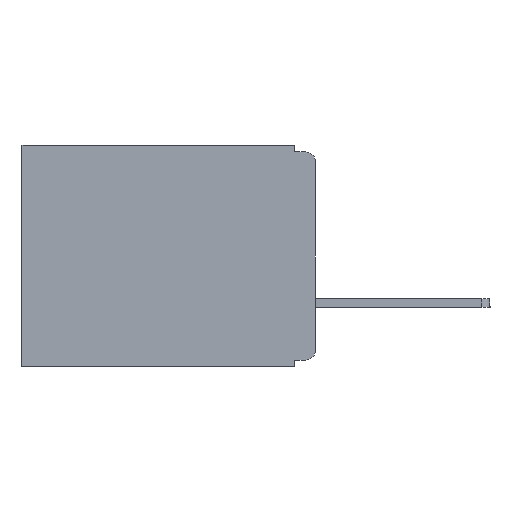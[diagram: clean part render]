
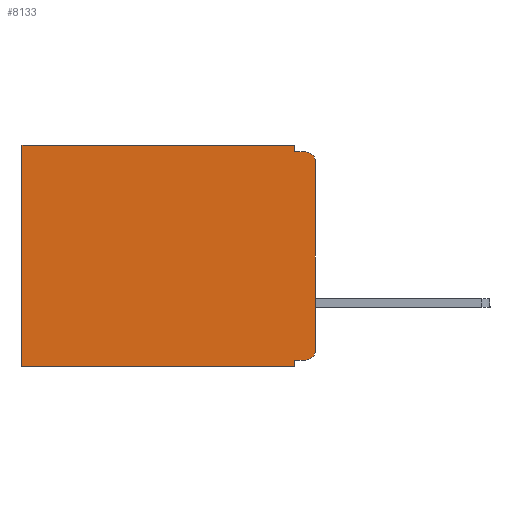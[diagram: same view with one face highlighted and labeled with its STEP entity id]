
A CAD part, left-side view. The second image highlights one B-rep face of the part: STEP entity #8133.
In plain terms, the highlighted planar face has unit normal (-1, 0, 0).
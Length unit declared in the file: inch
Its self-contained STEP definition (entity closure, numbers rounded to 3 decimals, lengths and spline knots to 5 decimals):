
#170 = CARTESIAN_POINT ( 'NONE',  ( 0.3, 0.437, -0.33 ) ) ;
#363 = CARTESIAN_POINT ( 'NONE',  ( 0.3, 0.031, -0.33 ) ) ;
#392 = CARTESIAN_POINT ( 'NONE',  ( 0.3, 0.031, 0. ) ) ;
#911 = ORIENTED_EDGE ( 'NONE', *, *, #4265, .T. ) ;
#1188 = VECTOR ( 'NONE', #18793, 39.37008 ) ;
#1235 = LINE ( 'NONE', #18116, #10656 ) ;
#1753 = DIRECTION ( 'NONE',  ( 0., 0., -1. ) ) ;
#1786 = LINE ( 'NONE', #16925, #1188 ) ;
#2096 = ORIENTED_EDGE ( 'NONE', *, *, #14630, .F. ) ;
#2279 = CARTESIAN_POINT ( 'NONE',  ( 0.3, 0.015, -0.025 ) ) ;
#2338 = CARTESIAN_POINT ( 'NONE',  ( 0.3, 0., -0.01 ) ) ;
#3538 = EDGE_CURVE ( 'NONE', #23070, #21568, #7645, .T. ) ;
#3553 = ORIENTED_EDGE ( 'NONE', *, *, #13994, .F. ) ;
#3990 = VECTOR ( 'NONE', #21921, 39.37008 ) ;
#4249 = VECTOR ( 'NONE', #19143, 39.37008 ) ;
#4265 = EDGE_CURVE ( 'NONE', #5508, #6899, #19861, .T. ) ;
#4614 = LINE ( 'NONE', #170, #9619 ) ;
#4848 = LINE ( 'NONE', #2338, #4249 ) ;
#5079 = AXIS2_PLACEMENT_3D ( 'NONE', #2279, #23373, #1753 ) ;
#5374 = EDGE_CURVE ( 'NONE', #23273, #9609, #4614, .T. ) ;
#5508 = VERTEX_POINT ( 'NONE', #17325 ) ;
#5601 = FACE_OUTER_BOUND ( 'NONE', #21836, .T. ) ;
#5902 = DIRECTION ( 'NONE',  ( 0., 0., -1. ) ) ;
#5985 = CIRCLE ( 'NONE', #12272, 0.015 ) ;
#6305 = CARTESIAN_POINT ( 'NONE',  ( 0.3, 0., -0.33 ) ) ;
#6521 = ORIENTED_EDGE ( 'NONE', *, *, #20665, .T. ) ;
#6614 = DIRECTION ( 'NONE',  ( -1., 0., 0. ) ) ;
#6899 = VERTEX_POINT ( 'NONE', #7066 ) ;
#7066 = CARTESIAN_POINT ( 'NONE',  ( 0.3, 0.015, -0.01 ) ) ;
#7314 = CARTESIAN_POINT ( 'NONE',  ( 0.3, 0.031, 0. ) ) ;
#7359 = ORIENTED_EDGE ( 'NONE', *, *, #3538, .F. ) ;
#7623 = DIRECTION ( 'NONE',  ( 0., 0., -1. ) ) ;
#7645 = LINE ( 'NONE', #392, #16981 ) ;
#7789 = CARTESIAN_POINT ( 'NONE',  ( 0.3, 0.031, -0.32 ) ) ;
#8133 = ADVANCED_FACE ( 'NONE', ( #5601 ), #17485, .F. ) ;
#8206 = DIRECTION ( 'NONE',  ( 0., 0., -1. ) ) ;
#8293 = ORIENTED_EDGE ( 'NONE', *, *, #12749, .F. ) ;
#8948 = CARTESIAN_POINT ( 'NONE',  ( 0.3, 0., 0. ) ) ;
#9609 = VERTEX_POINT ( 'NONE', #23721 ) ;
#9619 = VECTOR ( 'NONE', #7623, 39.37008 ) ;
#10656 = VECTOR ( 'NONE', #19975, 39.37008 ) ;
#11557 = CARTESIAN_POINT ( 'NONE',  ( 0.3, 0., -0.33 ) ) ;
#12272 = AXIS2_PLACEMENT_3D ( 'NONE', #17796, #6614, #19668 ) ;
#12738 = LINE ( 'NONE', #8948, #3990 ) ;
#12749 = EDGE_CURVE ( 'NONE', #16377, #22669, #16450, .T. ) ;
#13451 = EDGE_CURVE ( 'NONE', #23070, #23273, #12738, .T. ) ;
#13584 = AXIS2_PLACEMENT_3D ( 'NONE', #6305, #19371, #8206 ) ;
#13852 = VECTOR ( 'NONE', #5902, 39.37008 ) ;
#13994 = EDGE_CURVE ( 'NONE', #21568, #6899, #4848, .T. ) ;
#14432 = LINE ( 'NONE', #11557, #13852 ) ;
#14630 = EDGE_CURVE ( 'NONE', #5508, #19180, #14432, .T. ) ;
#14648 = ORIENTED_EDGE ( 'NONE', *, *, #15454, .F. ) ;
#15367 = CARTESIAN_POINT ( 'NONE',  ( 0.3, 0.437, 0. ) ) ;
#15454 = EDGE_CURVE ( 'NONE', #22669, #9609, #1235, .T. ) ;
#16316 = EDGE_CURVE ( 'NONE', #19260, #16377, #1786, .T. ) ;
#16377 = VERTEX_POINT ( 'NONE', #7789 ) ;
#16410 = ORIENTED_EDGE ( 'NONE', *, *, #5374, .T. ) ;
#16450 = LINE ( 'NONE', #18084, #21387 ) ;
#16925 = CARTESIAN_POINT ( 'NONE',  ( 0.3, 0., -0.32 ) ) ;
#16981 = VECTOR ( 'NONE', #17704, 39.37008 ) ;
#17325 = CARTESIAN_POINT ( 'NONE',  ( 0.3, 0., -0.025 ) ) ;
#17485 = PLANE ( 'NONE',  #13584 ) ;
#17704 = DIRECTION ( 'NONE',  ( 0., 0., -1. ) ) ;
#17796 = CARTESIAN_POINT ( 'NONE',  ( 0.3, 0.015, -0.305 ) ) ;
#18084 = CARTESIAN_POINT ( 'NONE',  ( 0.3, 0.031, -0.33 ) ) ;
#18116 = CARTESIAN_POINT ( 'NONE',  ( 0.3, 0., -0.33 ) ) ;
#18793 = DIRECTION ( 'NONE',  ( 0., 1., 0. ) ) ;
#19143 = DIRECTION ( 'NONE',  ( 0., -1., 0. ) ) ;
#19180 = VERTEX_POINT ( 'NONE', #21772 ) ;
#19260 = VERTEX_POINT ( 'NONE', #22008 ) ;
#19371 = DIRECTION ( 'NONE',  ( 1., 0., 0. ) ) ;
#19668 = DIRECTION ( 'NONE',  ( 0., 0., -1. ) ) ;
#19861 = CIRCLE ( 'NONE', #5079, 0.015 ) ;
#19975 = DIRECTION ( 'NONE',  ( 0., 1., 0. ) ) ;
#20665 = EDGE_CURVE ( 'NONE', #19260, #19180, #5985, .T. ) ;
#21053 = ORIENTED_EDGE ( 'NONE', *, *, #13451, .T. ) ;
#21375 = ORIENTED_EDGE ( 'NONE', *, *, #16316, .F. ) ;
#21387 = VECTOR ( 'NONE', #21792, 39.37008 ) ;
#21568 = VERTEX_POINT ( 'NONE', #22671 ) ;
#21772 = CARTESIAN_POINT ( 'NONE',  ( 0.3, 0., -0.305 ) ) ;
#21792 = DIRECTION ( 'NONE',  ( 0., 0., -1. ) ) ;
#21836 = EDGE_LOOP ( 'NONE', ( #2096, #911, #3553, #7359, #21053, #16410, #14648, #8293, #21375, #6521 ) ) ;
#21921 = DIRECTION ( 'NONE',  ( 0., 1., 0. ) ) ;
#22008 = CARTESIAN_POINT ( 'NONE',  ( 0.3, 0.015, -0.32 ) ) ;
#22669 = VERTEX_POINT ( 'NONE', #363 ) ;
#22671 = CARTESIAN_POINT ( 'NONE',  ( 0.3, 0.031, -0.01 ) ) ;
#23070 = VERTEX_POINT ( 'NONE', #7314 ) ;
#23273 = VERTEX_POINT ( 'NONE', #15367 ) ;
#23373 = DIRECTION ( 'NONE',  ( -1., 0., 0. ) ) ;
#23721 = CARTESIAN_POINT ( 'NONE',  ( 0.3, 0.437, -0.33 ) ) ;
